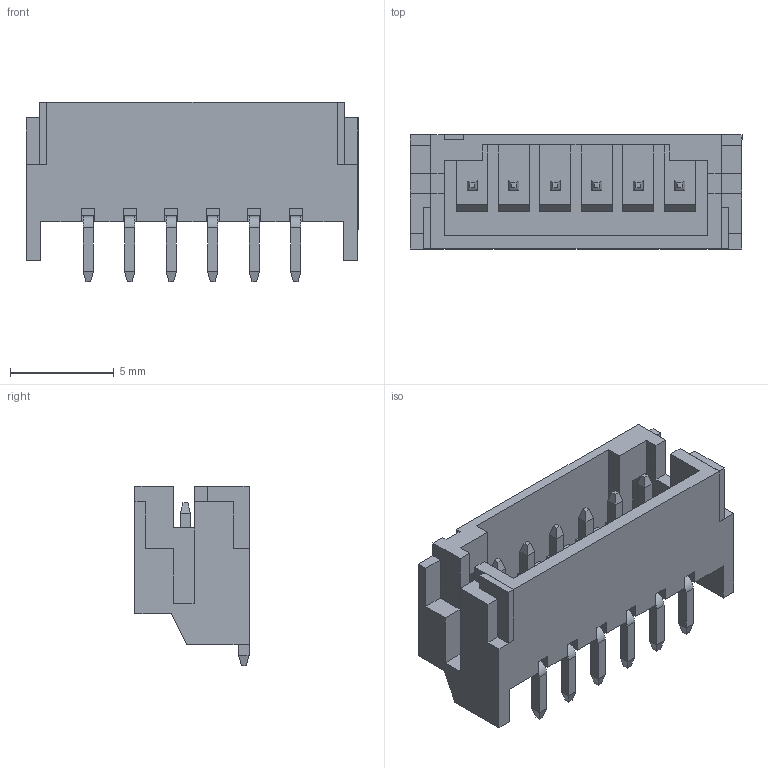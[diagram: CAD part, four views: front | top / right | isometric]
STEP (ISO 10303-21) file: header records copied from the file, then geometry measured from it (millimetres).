
FILE_DESCRIPTION (( 'STEP AP203' ), '1' );
FILE_NAME ('140-506-417-060.STEP', '2020-03-31T20:21:01', ( '' ), ( '' ), 'SwSTEP 2.0', 'SolidWorks 2016', '' );
FILE_SCHEMA (( 'CONFIG_CONTROL_DESIGN' ));
Length unit declared in the file: millimetre
Products named in the file (4): 140-506-417-060; RA SMT Contact; RA SMT Housing_506; RA SMT Pad
Assembly tree (9 placements, depth 2):
  140-506-417-060
    RA SMT Housing_506
    RA SMT Contact  x6
    RA SMT Pad  x2
Bounding box: 16 x 5.5 x 8.65 mm (x, y, z)
Volume: 235 mm3; surface area: 862 mm2
Topology: 9 solids, 9 shells, 356 faces, 880 edges, 538 vertices
Faces by surface type: plane 332, cylinder 24
Entity records: 6970 total; most frequent: CARTESIAN_POINT 1150, ORIENTED_EDGE 1136, DIRECTION 1000, EDGE_CURVE 568, LINE 560, VECTOR 560, VERTEX_POINT 370, AXIS2_PLACEMENT_3D 220
